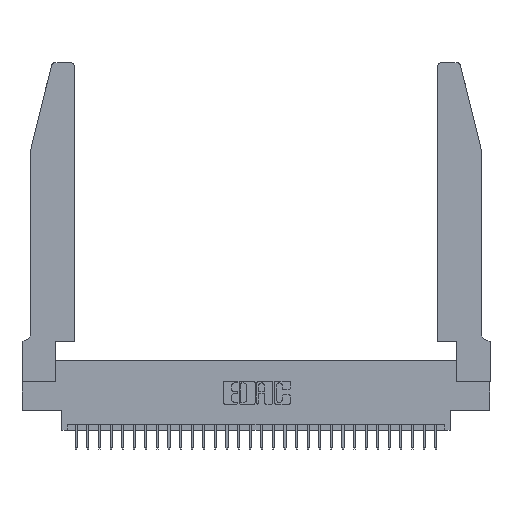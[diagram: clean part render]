
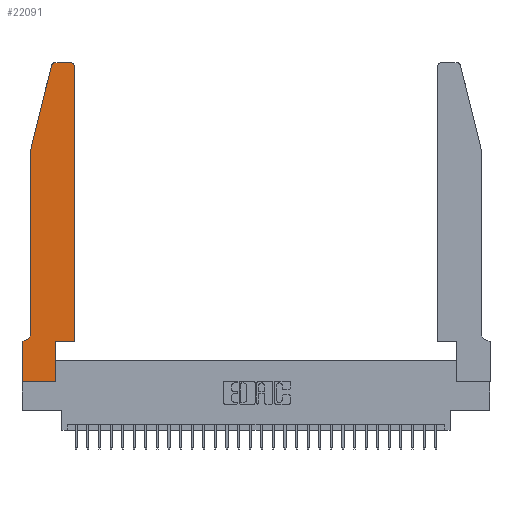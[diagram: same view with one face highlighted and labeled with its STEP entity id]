
A CAD part, top view. The second image highlights one B-rep face of the part: STEP entity #22091.
In plain terms, the highlighted planar face has unit normal (0, 0, 1).
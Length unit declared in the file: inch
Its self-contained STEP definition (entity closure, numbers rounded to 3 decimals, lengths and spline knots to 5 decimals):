
#16 = DIRECTION ( 'NONE',  ( 1., 0., 0. ) ) ;
#24 = DIRECTION ( 'NONE',  ( 0., -1., 0. ) ) ;
#58 = DIRECTION ( 'NONE',  ( 1., 0., 0. ) ) ;
#137 = CARTESIAN_POINT ( 'NONE',  ( 0.4505, 2.72, 0.37 ) ) ;
#348 = AXIS2_PLACEMENT_3D ( 'NONE', #22806, #8299, #25256 ) ;
#1376 = CARTESIAN_POINT ( 'NONE',  ( 0.2865, 0.35, 0.37 ) ) ;
#1401 = ORIENTED_EDGE ( 'NONE', *, *, #23888, .T. ) ;
#1458 = CARTESIAN_POINT ( 'NONE',  ( 0.284, 2.72, 0.37 ) ) ;
#1853 = EDGE_CURVE ( 'NONE', #27912, #28333, #27358, .T. ) ;
#2053 = CARTESIAN_POINT ( 'NONE',  ( 0.4505, 0.35, 0.37 ) ) ;
#2504 = VECTOR ( 'NONE', #24, 39.37008 ) ;
#2675 = ORIENTED_EDGE ( 'NONE', *, *, #26124, .T. ) ;
#3918 = DIRECTION ( 'NONE',  ( 1., 0., 0. ) ) ;
#4013 = CARTESIAN_POINT ( 'NONE',  ( 0.0055, 0.35, 0.37 ) ) ;
#4660 = VERTEX_POINT ( 'NONE', #19118 ) ;
#6156 = PLANE ( 'NONE',  #26777 ) ;
#6389 = FACE_OUTER_BOUND ( 'NONE', #14695, .T. ) ;
#6554 = EDGE_CURVE ( 'NONE', #28333, #26162, #14523, .T. ) ;
#6934 = CIRCLE ( 'NONE', #8629, 0.03 ) ;
#7340 = LINE ( 'NONE', #1376, #21019 ) ;
#8040 = VECTOR ( 'NONE', #26258, 39.37008 ) ;
#8299 = DIRECTION ( 'NONE',  ( 0., 0., -1. ) ) ;
#8364 = LINE ( 'NONE', #14653, #20500 ) ;
#8480 = LINE ( 'NONE', #15496, #14204 ) ;
#8517 = VERTEX_POINT ( 'NONE', #15634 ) ;
#8613 = DIRECTION ( 'NONE',  ( 1., 0., 0. ) ) ;
#8629 = AXIS2_PLACEMENT_3D ( 'NONE', #29130, #14721, #58 ) ;
#9257 = VERTEX_POINT ( 'NONE', #27474 ) ;
#10798 = CARTESIAN_POINT ( 'NONE',  ( 0.4505, 0.35, 0.37 ) ) ;
#11611 = VECTOR ( 'NONE', #16, 39.37008 ) ;
#12235 = ORIENTED_EDGE ( 'NONE', *, *, #24781, .T. ) ;
#13386 = CIRCLE ( 'NONE', #348, 0.07 ) ;
#13414 = VERTEX_POINT ( 'NONE', #4013 ) ;
#13629 = CARTESIAN_POINT ( 'NONE',  ( 0.0755, 0.42, 0.37 ) ) ;
#13630 = EDGE_CURVE ( 'NONE', #9257, #8517, #30867, .T. ) ;
#13698 = VERTEX_POINT ( 'NONE', #26781 ) ;
#13825 = AXIS2_PLACEMENT_3D ( 'NONE', #1458, #18520, #3918 ) ;
#13839 = CARTESIAN_POINT ( 'NONE',  ( 0., 0.35, 0.37 ) ) ;
#14204 = VECTOR ( 'NONE', #25197, 39.37008 ) ;
#14514 = ORIENTED_EDGE ( 'NONE', *, *, #19100, .T. ) ;
#14523 = LINE ( 'NONE', #2053, #8040 ) ;
#14537 = EDGE_CURVE ( 'NONE', #8517, #27912, #7340, .T. ) ;
#14653 = CARTESIAN_POINT ( 'NONE',  ( 0., 0., 0.37 ) ) ;
#14683 = LINE ( 'NONE', #29242, #26731 ) ;
#14695 = EDGE_LOOP ( 'NONE', ( #20925, #18374, #14514, #2675, #1401, #28373, #12235, #16824, #15719, #27931, #25328, #17069 ) ) ;
#14721 = DIRECTION ( 'NONE',  ( 0., 0., 1. ) ) ;
#14835 = EDGE_CURVE ( 'NONE', #26162, #23264, #6934, .T. ) ;
#15314 = VECTOR ( 'NONE', #20657, 39.37008 ) ;
#15496 = CARTESIAN_POINT ( 'NONE',  ( 0.0755, 2., 0.37 ) ) ;
#15634 = CARTESIAN_POINT ( 'NONE',  ( 0.2865, 0., 0.37 ) ) ;
#15719 = ORIENTED_EDGE ( 'NONE', *, *, #14537, .T. ) ;
#15722 = VERTEX_POINT ( 'NONE', #25536 ) ;
#16824 = ORIENTED_EDGE ( 'NONE', *, *, #13630, .T. ) ;
#17069 = ORIENTED_EDGE ( 'NONE', *, *, #14835, .T. ) ;
#17255 = DIRECTION ( 'NONE',  ( -1., 0., 0. ) ) ;
#18281 = CARTESIAN_POINT ( 'NONE',  ( 0., 0.35, 0.37 ) ) ;
#18356 = CARTESIAN_POINT ( 'NONE',  ( 0.4505, 0.35, 0.37 ) ) ;
#18374 = ORIENTED_EDGE ( 'NONE', *, *, #30211, .T. ) ;
#18520 = DIRECTION ( 'NONE',  ( 0., 0., 1. ) ) ;
#19100 = EDGE_CURVE ( 'NONE', #13698, #15722, #8480, .T. ) ;
#19118 = CARTESIAN_POINT ( 'NONE',  ( 0.284, 2.75, 0.37 ) ) ;
#19332 = DIRECTION ( 'NONE',  ( -1., 0., 0. ) ) ;
#20113 = CARTESIAN_POINT ( 'NONE',  ( 0.4205, 2.75, 0.37 ) ) ;
#20500 = VECTOR ( 'NONE', #21921, 39.37008 ) ;
#20657 = DIRECTION ( 'NONE',  ( 1., 0., 0. ) ) ;
#20925 = ORIENTED_EDGE ( 'NONE', *, *, #28209, .T. ) ;
#21019 = VECTOR ( 'NONE', #25502, 39.37008 ) ;
#21921 = DIRECTION ( 'NONE',  ( 0., -1., 0. ) ) ;
#22037 = LINE ( 'NONE', #24077, #29951 ) ;
#22091 = ADVANCED_FACE ( 'NONE', ( #6389 ), #6156, .T. ) ;
#22237 = VERTEX_POINT ( 'NONE', #13839 ) ;
#22806 = CARTESIAN_POINT ( 'NONE',  ( 0.0055, 0.42, 0.37 ) ) ;
#23118 = DIRECTION ( 'NONE',  ( 0., 0., 1. ) ) ;
#23264 = VERTEX_POINT ( 'NONE', #20113 ) ;
#23888 = EDGE_CURVE ( 'NONE', #31120, #13414, #13386, .T. ) ;
#24077 = CARTESIAN_POINT ( 'NONE',  ( 0.0755, 0.35, 0.37 ) ) ;
#24245 = EDGE_CURVE ( 'NONE', #13414, #22237, #22037, .T. ) ;
#24781 = EDGE_CURVE ( 'NONE', #22237, #9257, #8364, .T. ) ;
#25197 = DIRECTION ( 'NONE',  ( -0.239, -0.971, 0. ) ) ;
#25256 = DIRECTION ( 'NONE',  ( -1., 0., 0. ) ) ;
#25328 = ORIENTED_EDGE ( 'NONE', *, *, #6554, .T. ) ;
#25502 = DIRECTION ( 'NONE',  ( 0., 1., 0. ) ) ;
#25536 = CARTESIAN_POINT ( 'NONE',  ( 0.0755, 2., 0.37 ) ) ;
#26124 = EDGE_CURVE ( 'NONE', #15722, #31120, #27573, .T. ) ;
#26162 = VERTEX_POINT ( 'NONE', #137 ) ;
#26258 = DIRECTION ( 'NONE',  ( 0., 1., 0. ) ) ;
#26731 = VECTOR ( 'NONE', #17255, 39.37008 ) ;
#26777 = AXIS2_PLACEMENT_3D ( 'NONE', #18281, #23118, #8613 ) ;
#26781 = CARTESIAN_POINT ( 'NONE',  ( 0.25487, 2.72718, 0.37 ) ) ;
#27358 = LINE ( 'NONE', #18356, #15314 ) ;
#27474 = CARTESIAN_POINT ( 'NONE',  ( 0., 0., 0.37 ) ) ;
#27573 = LINE ( 'NONE', #29087, #2504 ) ;
#27912 = VERTEX_POINT ( 'NONE', #28219 ) ;
#27931 = ORIENTED_EDGE ( 'NONE', *, *, #1853, .T. ) ;
#28209 = EDGE_CURVE ( 'NONE', #23264, #4660, #14683, .T. ) ;
#28219 = CARTESIAN_POINT ( 'NONE',  ( 0.2865, 0.35, 0.37 ) ) ;
#28333 = VERTEX_POINT ( 'NONE', #10798 ) ;
#28373 = ORIENTED_EDGE ( 'NONE', *, *, #24245, .T. ) ;
#28517 = CIRCLE ( 'NONE', #13825, 0.03 ) ;
#29083 = CARTESIAN_POINT ( 'NONE',  ( 0., 0., 0.37 ) ) ;
#29087 = CARTESIAN_POINT ( 'NONE',  ( 0.0755, 2., 0.37 ) ) ;
#29130 = CARTESIAN_POINT ( 'NONE',  ( 0.4205, 2.72, 0.37 ) ) ;
#29242 = CARTESIAN_POINT ( 'NONE',  ( 0.2605, 2.75, 0.37 ) ) ;
#29951 = VECTOR ( 'NONE', #19332, 39.37008 ) ;
#30211 = EDGE_CURVE ( 'NONE', #4660, #13698, #28517, .T. ) ;
#30867 = LINE ( 'NONE', #29083, #11611 ) ;
#31120 = VERTEX_POINT ( 'NONE', #13629 ) ;
